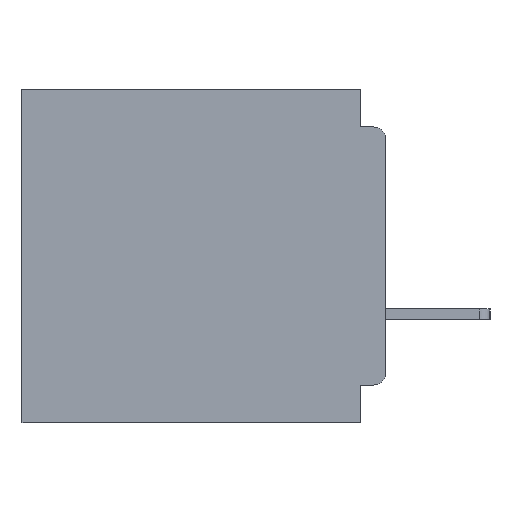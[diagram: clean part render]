
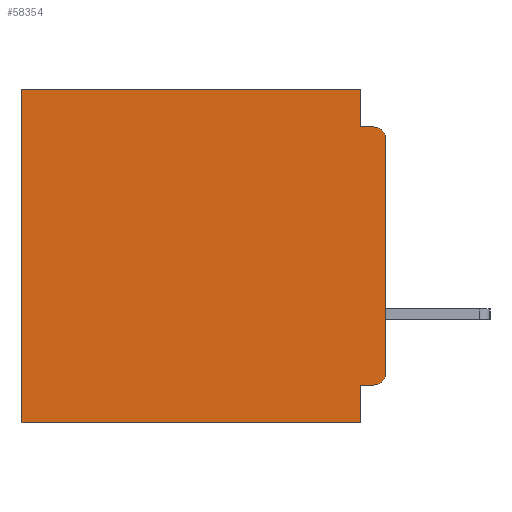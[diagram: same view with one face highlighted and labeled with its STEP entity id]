
A CAD part, left-side view. The second image highlights one B-rep face of the part: STEP entity #58354.
In plain terms, the highlighted planar face has unit normal (-1, 0, 0).
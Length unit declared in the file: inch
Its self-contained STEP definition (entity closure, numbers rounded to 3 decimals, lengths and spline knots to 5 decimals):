
#1055 = CARTESIAN_POINT ( 'NONE',  ( 0.3, 0.031, -0.4 ) ) ;
#1487 = DIRECTION ( 'NONE',  ( 0., 0., -1. ) ) ;
#1689 = LINE ( 'NONE', #52722, #55864 ) ;
#2869 = VERTEX_POINT ( 'NONE', #65563 ) ;
#3268 = LINE ( 'NONE', #18743, #29438 ) ;
#5754 = LINE ( 'NONE', #11660, #18054 ) ;
#5862 = CARTESIAN_POINT ( 'NONE',  ( 0.3, 0., -0.4 ) ) ;
#7278 = CARTESIAN_POINT ( 'NONE',  ( 0.3, 0., -0.4 ) ) ;
#7675 = DIRECTION ( 'NONE',  ( 0., 1., 0. ) ) ;
#7879 = EDGE_CURVE ( 'NONE', #62902, #54532, #57572, .T. ) ;
#10472 = EDGE_CURVE ( 'NONE', #16808, #14756, #1689, .T. ) ;
#10709 = ORIENTED_EDGE ( 'NONE', *, *, #31002, .F. ) ;
#11108 = DIRECTION ( 'NONE',  ( 0., 0., -1. ) ) ;
#11588 = CARTESIAN_POINT ( 'NONE',  ( 0.3, 0.015, -0.34 ) ) ;
#11660 = CARTESIAN_POINT ( 'NONE',  ( 0.3, 0., -0.045 ) ) ;
#12490 = DIRECTION ( 'NONE',  ( 0., 0., -1. ) ) ;
#13514 = VERTEX_POINT ( 'NONE', #53742 ) ;
#14193 = ORIENTED_EDGE ( 'NONE', *, *, #61219, .F. ) ;
#14756 = VERTEX_POINT ( 'NONE', #49231 ) ;
#15968 = DIRECTION ( 'NONE',  ( 0., 0., -1. ) ) ;
#16286 = EDGE_CURVE ( 'NONE', #53670, #16808, #3268, .T. ) ;
#16391 = CARTESIAN_POINT ( 'NONE',  ( 0.3, 0.015, -0.06 ) ) ;
#16808 = VERTEX_POINT ( 'NONE', #38374 ) ;
#16876 = DIRECTION ( 'NONE',  ( 0., 0., -1. ) ) ;
#17678 = ORIENTED_EDGE ( 'NONE', *, *, #23787, .T. ) ;
#17876 = CARTESIAN_POINT ( 'NONE',  ( 0.3, 0.031, 0. ) ) ;
#18054 = VECTOR ( 'NONE', #53718, 39.37008 ) ;
#18743 = CARTESIAN_POINT ( 'NONE',  ( 0.3, 0., 0. ) ) ;
#20032 = VECTOR ( 'NONE', #1487, 39.37008 ) ;
#21063 = ORIENTED_EDGE ( 'NONE', *, *, #16286, .T. ) ;
#21651 = DIRECTION ( 'NONE',  ( 0., 0., -1. ) ) ;
#23787 = EDGE_CURVE ( 'NONE', #62902, #53687, #24276, .T. ) ;
#24276 = CIRCLE ( 'NONE', #67239, 0.015 ) ;
#24292 = VECTOR ( 'NONE', #12490, 39.37008 ) ;
#24816 = ORIENTED_EDGE ( 'NONE', *, *, #66434, .F. ) ;
#25563 = EDGE_CURVE ( 'NONE', #64282, #47815, #45426, .T. ) ;
#27232 = CARTESIAN_POINT ( 'NONE',  ( 0.3, 0.015, -0.355 ) ) ;
#27259 = ORIENTED_EDGE ( 'NONE', *, *, #10472, .T. ) ;
#27295 = AXIS2_PLACEMENT_3D ( 'NONE', #16391, #53159, #21651 ) ;
#27376 = ORIENTED_EDGE ( 'NONE', *, *, #56984, .F. ) ;
#29264 = DIRECTION ( 'NONE',  ( 0., 1., 0. ) ) ;
#29438 = VECTOR ( 'NONE', #29264, 39.37008 ) ;
#31002 = EDGE_CURVE ( 'NONE', #64282, #53687, #63613, .T. ) ;
#37219 = PLANE ( 'NONE',  #48296 ) ;
#37384 = CARTESIAN_POINT ( 'NONE',  ( 0.3, 0.015, -0.045 ) ) ;
#37643 = DIRECTION ( 'NONE',  ( 0., 0., -1. ) ) ;
#37949 = EDGE_CURVE ( 'NONE', #54532, #13514, #55282, .T. ) ;
#38093 = CARTESIAN_POINT ( 'NONE',  ( 0.3, 0., -0.4 ) ) ;
#38374 = CARTESIAN_POINT ( 'NONE',  ( 0.3, 0.437, 0. ) ) ;
#38694 = DIRECTION ( 'NONE',  ( 0., 1., 0. ) ) ;
#39093 = CARTESIAN_POINT ( 'NONE',  ( 0.3, 0., -0.355 ) ) ;
#40245 = ORIENTED_EDGE ( 'NONE', *, *, #25563, .T. ) ;
#42160 = ORIENTED_EDGE ( 'NONE', *, *, #7879, .F. ) ;
#42575 = DIRECTION ( 'NONE',  ( 1., 0., 0. ) ) ;
#45426 = CIRCLE ( 'NONE', #27295, 0.015 ) ;
#46751 = EDGE_LOOP ( 'NONE', ( #10709, #40245, #24816, #27376, #21063, #27259, #14193, #48298, #42160, #17678 ) ) ;
#47815 = VERTEX_POINT ( 'NONE', #37384 ) ;
#48296 = AXIS2_PLACEMENT_3D ( 'NONE', #5862, #42575, #11108 ) ;
#48298 = ORIENTED_EDGE ( 'NONE', *, *, #37949, .F. ) ;
#48366 = DIRECTION ( 'NONE',  ( -1., 0., 0. ) ) ;
#49231 = CARTESIAN_POINT ( 'NONE',  ( 0.3, 0.437, -0.4 ) ) ;
#49259 = CARTESIAN_POINT ( 'NONE',  ( 0.3, 0.031, 0. ) ) ;
#50746 = LINE ( 'NONE', #7278, #63084 ) ;
#52722 = CARTESIAN_POINT ( 'NONE',  ( 0.3, 0.437, -0.4 ) ) ;
#53159 = DIRECTION ( 'NONE',  ( -1., 0., 0. ) ) ;
#53603 = CARTESIAN_POINT ( 'NONE',  ( 0.3, 0., -0.06 ) ) ;
#53670 = VERTEX_POINT ( 'NONE', #17876 ) ;
#53687 = VERTEX_POINT ( 'NONE', #65186 ) ;
#53718 = DIRECTION ( 'NONE',  ( 0., -1., 0. ) ) ;
#53742 = CARTESIAN_POINT ( 'NONE',  ( 0.3, 0.031, -0.4 ) ) ;
#53934 = LINE ( 'NONE', #49259, #24292 ) ;
#54532 = VERTEX_POINT ( 'NONE', #63258 ) ;
#55282 = LINE ( 'NONE', #1055, #58559 ) ;
#55864 = VECTOR ( 'NONE', #15968, 39.37008 ) ;
#56984 = EDGE_CURVE ( 'NONE', #53670, #2869, #53934, .T. ) ;
#57572 = LINE ( 'NONE', #39093, #66583 ) ;
#58354 = ADVANCED_FACE ( 'NONE', ( #62764 ), #37219, .F. ) ;
#58559 = VECTOR ( 'NONE', #37643, 39.37008 ) ;
#61219 = EDGE_CURVE ( 'NONE', #13514, #14756, #50746, .T. ) ;
#62764 = FACE_OUTER_BOUND ( 'NONE', #46751, .T. ) ;
#62902 = VERTEX_POINT ( 'NONE', #27232 ) ;
#63084 = VECTOR ( 'NONE', #38694, 39.37008 ) ;
#63258 = CARTESIAN_POINT ( 'NONE',  ( 0.3, 0.031, -0.355 ) ) ;
#63613 = LINE ( 'NONE', #38093, #20032 ) ;
#64282 = VERTEX_POINT ( 'NONE', #53603 ) ;
#65186 = CARTESIAN_POINT ( 'NONE',  ( 0.3, 0., -0.34 ) ) ;
#65563 = CARTESIAN_POINT ( 'NONE',  ( 0.3, 0.031, -0.045 ) ) ;
#66434 = EDGE_CURVE ( 'NONE', #2869, #47815, #5754, .T. ) ;
#66583 = VECTOR ( 'NONE', #7675, 39.37008 ) ;
#67239 = AXIS2_PLACEMENT_3D ( 'NONE', #11588, #48366, #16876 ) ;
